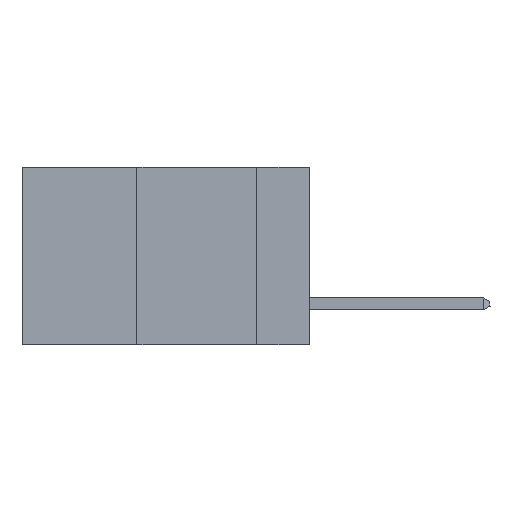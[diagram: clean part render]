
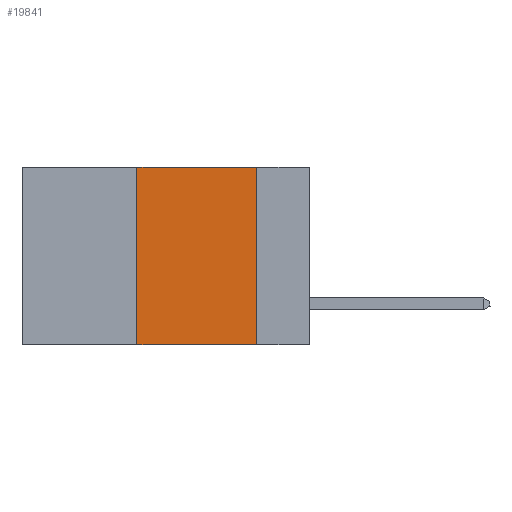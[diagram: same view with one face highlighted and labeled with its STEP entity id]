
A CAD part, left-side view. The second image highlights one B-rep face of the part: STEP entity #19841.
In plain terms, the highlighted planar face has unit normal (-1, 0, 0).
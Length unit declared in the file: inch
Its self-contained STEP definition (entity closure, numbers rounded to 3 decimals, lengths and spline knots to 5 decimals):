
#275 = AXIS2_PLACEMENT_3D ( 'NONE', #8363, #5072, #14950 ) ;
#846 = LINE ( 'NONE', #11374, #4158 ) ;
#1698 = EDGE_CURVE ( 'NONE', #14880, #17436, #8458, .T. ) ;
#3000 = EDGE_CURVE ( 'NONE', #7557, #14880, #8901, .T. ) ;
#3244 = DIRECTION ( 'NONE',  ( 0., -1., 0. ) ) ;
#4158 = VECTOR ( 'NONE', #11672, 39.37008 ) ;
#4332 = DIRECTION ( 'NONE',  ( 0., -1., 0. ) ) ;
#4933 = CARTESIAN_POINT ( 'NONE',  ( 0., 0.11, 0. ) ) ;
#5072 = DIRECTION ( 'NONE',  ( 1., 0., 0. ) ) ;
#6097 = ORIENTED_EDGE ( 'NONE', *, *, #12493, .T. ) ;
#7342 = CARTESIAN_POINT ( 'NONE',  ( 0., 0.6, 0. ) ) ;
#7557 = VERTEX_POINT ( 'NONE', #9921 ) ;
#8006 = CARTESIAN_POINT ( 'NONE',  ( 0., 0.36, 0. ) ) ;
#8363 = CARTESIAN_POINT ( 'NONE',  ( 0., 0.6, 0. ) ) ;
#8410 = EDGE_CURVE ( 'NONE', #17436, #17026, #846, .T. ) ;
#8458 = LINE ( 'NONE', #7342, #17934 ) ;
#8680 = CARTESIAN_POINT ( 'NONE',  ( 0., 0.6, -0.37 ) ) ;
#8901 = LINE ( 'NONE', #14038, #17105 ) ;
#9921 = CARTESIAN_POINT ( 'NONE',  ( 0., 0.36, -0.37 ) ) ;
#10083 = PLANE ( 'NONE',  #275 ) ;
#11374 = CARTESIAN_POINT ( 'NONE',  ( 0., 0.11, 0. ) ) ;
#11672 = DIRECTION ( 'NONE',  ( 0., 0., -1. ) ) ;
#12493 = EDGE_CURVE ( 'NONE', #7557, #17026, #20386, .T. ) ;
#13617 = CARTESIAN_POINT ( 'NONE',  ( 0., 0.11, -0.37 ) ) ;
#13894 = EDGE_LOOP ( 'NONE', ( #15490, #16589, #14929, #6097 ) ) ;
#14038 = CARTESIAN_POINT ( 'NONE',  ( 0., 0.36, 0. ) ) ;
#14880 = VERTEX_POINT ( 'NONE', #8006 ) ;
#14929 = ORIENTED_EDGE ( 'NONE', *, *, #3000, .F. ) ;
#14950 = DIRECTION ( 'NONE',  ( 0., 0., -1. ) ) ;
#15490 = ORIENTED_EDGE ( 'NONE', *, *, #8410, .F. ) ;
#16589 = ORIENTED_EDGE ( 'NONE', *, *, #1698, .F. ) ;
#16948 = FACE_OUTER_BOUND ( 'NONE', #13894, .T. ) ;
#17026 = VERTEX_POINT ( 'NONE', #13617 ) ;
#17105 = VECTOR ( 'NONE', #18759, 39.37008 ) ;
#17436 = VERTEX_POINT ( 'NONE', #4933 ) ;
#17934 = VECTOR ( 'NONE', #4332, 39.37008 ) ;
#18759 = DIRECTION ( 'NONE',  ( 0., 0., 1. ) ) ;
#19841 = ADVANCED_FACE ( 'NONE', ( #16948 ), #10083, .F. ) ;
#20386 = LINE ( 'NONE', #8680, #20901 ) ;
#20901 = VECTOR ( 'NONE', #3244, 39.37008 ) ;
